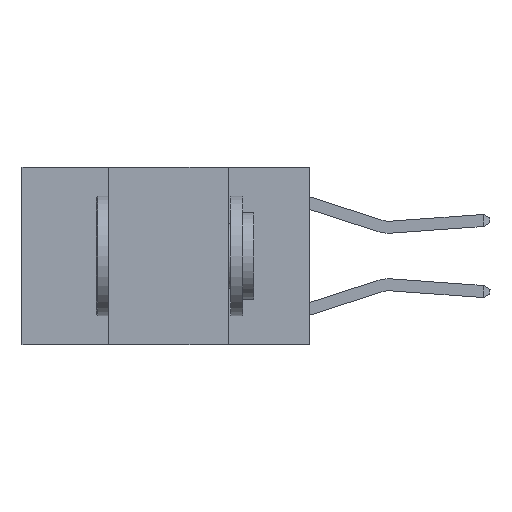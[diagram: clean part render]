
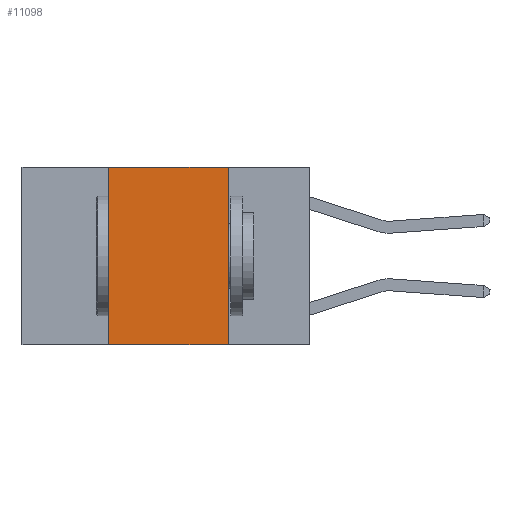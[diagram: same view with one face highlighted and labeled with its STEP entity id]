
A CAD part, left-side view. The second image highlights one B-rep face of the part: STEP entity #11098.
In plain terms, the highlighted planar face has unit normal (-1, 0, 0).
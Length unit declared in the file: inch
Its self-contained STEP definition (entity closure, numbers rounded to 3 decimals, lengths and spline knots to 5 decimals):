
#161 = VERTEX_POINT ( 'NONE', #13099 ) ;
#307 = EDGE_CURVE ( 'NONE', #12680, #5940, #797, .T. ) ;
#797 = LINE ( 'NONE', #6152, #11421 ) ;
#1010 = ORIENTED_EDGE ( 'NONE', *, *, #6531, .F. ) ;
#1269 = VECTOR ( 'NONE', #7857, 39.37008 ) ;
#1426 = LINE ( 'NONE', #9661, #12011 ) ;
#2512 = DIRECTION ( 'NONE',  ( 0., 0., 1. ) ) ;
#2571 = CARTESIAN_POINT ( 'NONE',  ( 0., 0.6, 0. ) ) ;
#2737 = CARTESIAN_POINT ( 'NONE',  ( 0., 0.6, -0.37 ) ) ;
#4074 = LINE ( 'NONE', #2737, #1269 ) ;
#4510 = ORIENTED_EDGE ( 'NONE', *, *, #307, .F. ) ;
#4667 = DIRECTION ( 'NONE',  ( 1., 0., 0. ) ) ;
#5489 = DIRECTION ( 'NONE',  ( 0., 0., -1. ) ) ;
#5940 = VERTEX_POINT ( 'NONE', #12769 ) ;
#6152 = CARTESIAN_POINT ( 'NONE',  ( 0., 0.6, 0. ) ) ;
#6492 = AXIS2_PLACEMENT_3D ( 'NONE', #2571, #4667, #11752 ) ;
#6531 = EDGE_CURVE ( 'NONE', #8454, #12680, #1426, .T. ) ;
#6906 = VECTOR ( 'NONE', #5489, 39.37008 ) ;
#6966 = EDGE_CURVE ( 'NONE', #5940, #161, #12316, .T. ) ;
#7023 = DIRECTION ( 'NONE',  ( 0., -1., 0. ) ) ;
#7749 = CARTESIAN_POINT ( 'NONE',  ( 0., 0.42, 0. ) ) ;
#7857 = DIRECTION ( 'NONE',  ( 0., -1., 0. ) ) ;
#7900 = ORIENTED_EDGE ( 'NONE', *, *, #9945, .T. ) ;
#8454 = VERTEX_POINT ( 'NONE', #9800 ) ;
#8527 = CARTESIAN_POINT ( 'NONE',  ( 0., 0.17, 0. ) ) ;
#9074 = ORIENTED_EDGE ( 'NONE', *, *, #6966, .F. ) ;
#9661 = CARTESIAN_POINT ( 'NONE',  ( 0., 0.42, 0. ) ) ;
#9800 = CARTESIAN_POINT ( 'NONE',  ( 0., 0.42, -0.37 ) ) ;
#9945 = EDGE_CURVE ( 'NONE', #8454, #161, #4074, .T. ) ;
#10760 = PLANE ( 'NONE',  #6492 ) ;
#11098 = ADVANCED_FACE ( 'NONE', ( #11350 ), #10760, .F. ) ;
#11350 = FACE_OUTER_BOUND ( 'NONE', #13229, .T. ) ;
#11421 = VECTOR ( 'NONE', #7023, 39.37008 ) ;
#11752 = DIRECTION ( 'NONE',  ( 0., 0., -1. ) ) ;
#12011 = VECTOR ( 'NONE', #2512, 39.37008 ) ;
#12316 = LINE ( 'NONE', #8527, #6906 ) ;
#12680 = VERTEX_POINT ( 'NONE', #7749 ) ;
#12769 = CARTESIAN_POINT ( 'NONE',  ( 0., 0.17, 0. ) ) ;
#13099 = CARTESIAN_POINT ( 'NONE',  ( 0., 0.17, -0.37 ) ) ;
#13229 = EDGE_LOOP ( 'NONE', ( #9074, #4510, #1010, #7900 ) ) ;
